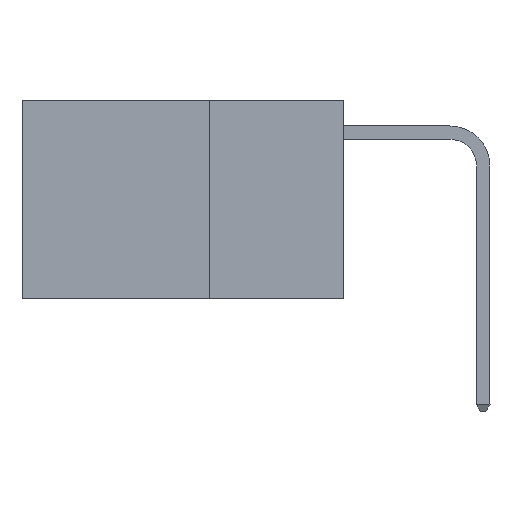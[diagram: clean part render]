
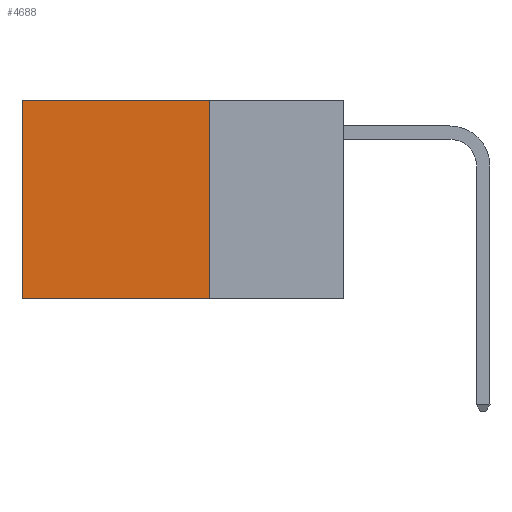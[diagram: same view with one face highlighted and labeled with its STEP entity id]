
A CAD part, left-side view. The second image highlights one B-rep face of the part: STEP entity #4688.
In plain terms, the highlighted planar face has unit normal (-1, 0, 0).
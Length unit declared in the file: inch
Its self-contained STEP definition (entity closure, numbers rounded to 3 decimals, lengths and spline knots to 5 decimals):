
#51 = EDGE_CURVE ( 'NONE', #10432, #5441, #11356, .T. ) ;
#281 = VERTEX_POINT ( 'NONE', #3972 ) ;
#945 = VECTOR ( 'NONE', #1082, 39.37008 ) ;
#1052 = CARTESIAN_POINT ( 'NONE',  ( 0.2625, 0.25, -0.37 ) ) ;
#1082 = DIRECTION ( 'NONE',  ( 0., 1., 0. ) ) ;
#1483 = DIRECTION ( 'NONE',  ( 0., 0., -1. ) ) ;
#1489 = DIRECTION ( 'NONE',  ( 1., 0., 0. ) ) ;
#1499 = CARTESIAN_POINT ( 'NONE',  ( 0.2625, 0.25, 0. ) ) ;
#1529 = PLANE ( 'NONE',  #5659 ) ;
#2653 = VECTOR ( 'NONE', #3658, 39.37008 ) ;
#2855 = CARTESIAN_POINT ( 'NONE',  ( 0.2625, 0.6, 0. ) ) ;
#2938 = LINE ( 'NONE', #11499, #2653 ) ;
#3166 = VERTEX_POINT ( 'NONE', #10947 ) ;
#3658 = DIRECTION ( 'NONE',  ( 0., 0., -1. ) ) ;
#3972 = CARTESIAN_POINT ( 'NONE',  ( 0.2625, 0.25, -0.37 ) ) ;
#3994 = ORIENTED_EDGE ( 'NONE', *, *, #10913, .F. ) ;
#4688 = ADVANCED_FACE ( 'NONE', ( #5493 ), #1529, .F. ) ;
#4776 = VECTOR ( 'NONE', #9351, 39.37008 ) ;
#4789 = EDGE_CURVE ( 'NONE', #281, #5441, #8914, .T. ) ;
#5194 = ORIENTED_EDGE ( 'NONE', *, *, #51, .T. ) ;
#5441 = VERTEX_POINT ( 'NONE', #7114 ) ;
#5493 = FACE_OUTER_BOUND ( 'NONE', #10512, .T. ) ;
#5659 = AXIS2_PLACEMENT_3D ( 'NONE', #1499, #1489, #1483 ) ;
#6333 = ORIENTED_EDGE ( 'NONE', *, *, #4789, .F. ) ;
#7114 = CARTESIAN_POINT ( 'NONE',  ( 0.2625, 0.6, -0.37 ) ) ;
#8564 = EDGE_CURVE ( 'NONE', #3166, #10432, #9710, .T. ) ;
#8826 = DIRECTION ( 'NONE',  ( 0., 0., -1. ) ) ;
#8852 = VECTOR ( 'NONE', #8826, 39.37008 ) ;
#8914 = LINE ( 'NONE', #1052, #945 ) ;
#8947 = CARTESIAN_POINT ( 'NONE',  ( 0.2625, 0.6, 0. ) ) ;
#9351 = DIRECTION ( 'NONE',  ( 0., 1., 0. ) ) ;
#9710 = LINE ( 'NONE', #12142, #4776 ) ;
#10432 = VERTEX_POINT ( 'NONE', #2855 ) ;
#10512 = EDGE_LOOP ( 'NONE', ( #5194, #6333, #3994, #10663 ) ) ;
#10663 = ORIENTED_EDGE ( 'NONE', *, *, #8564, .T. ) ;
#10913 = EDGE_CURVE ( 'NONE', #3166, #281, #2938, .T. ) ;
#10947 = CARTESIAN_POINT ( 'NONE',  ( 0.2625, 0.25, 0. ) ) ;
#11356 = LINE ( 'NONE', #8947, #8852 ) ;
#11499 = CARTESIAN_POINT ( 'NONE',  ( 0.2625, 0.25, 0. ) ) ;
#12142 = CARTESIAN_POINT ( 'NONE',  ( 0.2625, 0.25, 0. ) ) ;
